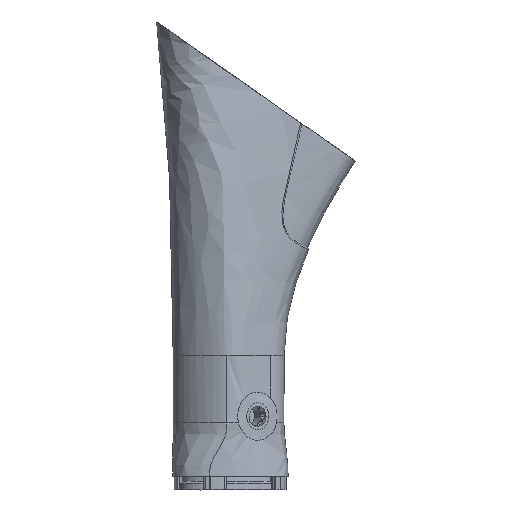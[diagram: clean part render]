
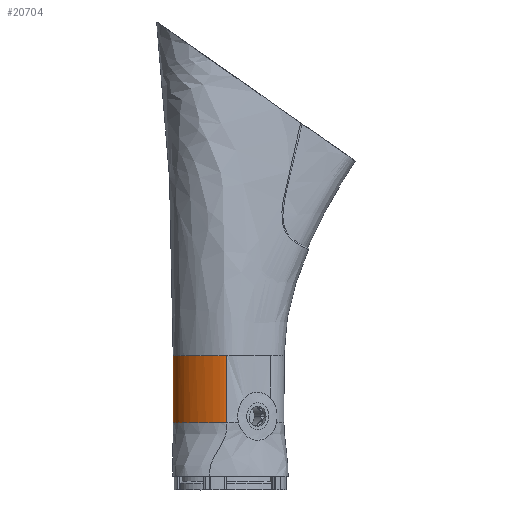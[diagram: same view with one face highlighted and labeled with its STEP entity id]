
A CAD part, left-side view. The second image highlights one B-rep face of the part: STEP entity #20704.
In plain terms, the highlighted free-form (B-spline) face has degree [3, 1] with [6, 2] control points.
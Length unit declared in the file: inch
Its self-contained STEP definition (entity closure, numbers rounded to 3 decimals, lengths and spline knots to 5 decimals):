
#194 = CARTESIAN_POINT ( 'NONE',  ( 0.05, 0.69, 1.5 ) ) ;
#334 = CARTESIAN_POINT ( 'NONE',  ( -0.89443, -0.31, 0.25 ) ) ;
#439 = CARTESIAN_POINT ( 'NONE',  ( 0.89443, -0.31, -3.73696 ) ) ;
#663 = ORIENTED_EDGE ( 'NONE', *, *, #16492, .F. ) ;
#770 = CARTESIAN_POINT ( 'NONE',  ( 0.89443, -0.31, 0.25 ) ) ;
#801 = CARTESIAN_POINT ( 'NONE',  ( 0.89443, -0.085, 0.25 ) ) ;
#976 = CARTESIAN_POINT ( 'NONE',  ( 0.89443, -0.085, 0.25 ) ) ;
#1501 = VERTEX_POINT ( 'NONE', #1584 ) ;
#1584 = CARTESIAN_POINT ( 'NONE',  ( 0.89443, -0.31, 1.5 ) ) ;
#1792 = DIRECTION ( 'NONE',  ( 0., 0., 1. ) ) ;
#2151 = LINE ( 'NONE', #5636, #6330 ) ;
#3338 = CARTESIAN_POINT ( 'NONE',  ( -0.89443, -0.31, 1.5 ) ) ;
#3463 = CARTESIAN_POINT ( 'NONE',  ( 0.89443, -0.31, 1.5 ) ) ;
#3648 = EDGE_CURVE ( 'NONE', #6380, #21719, #2151, .T. ) ;
#4115 = ORIENTED_EDGE ( 'NONE', *, *, #3648, .T. ) ;
#4367 = CARTESIAN_POINT ( 'NONE',  ( 0.51556, 0.69646, 0.25 ) ) ;
#5636 = CARTESIAN_POINT ( 'NONE',  ( -0.89443, -0.31, -3.73696 ) ) ;
#5839 = CARTESIAN_POINT ( 'NONE',  ( -0.89443, -0.31, 0.25 ) ) ;
#5906 = CARTESIAN_POINT ( 'NONE',  ( -0.55, 0.62542, 1.5 ) ) ;
#6310 = CARTESIAN_POINT ( 'NONE',  ( -0.89443, -0.085, 1.5 ) ) ;
#6330 = VECTOR ( 'NONE', #9129, 39.37008 ) ;
#6380 = VERTEX_POINT ( 'NONE', #334 ) ;
#6917 = EDGE_CURVE ( 'NONE', #1501, #19373, #16355, .T. ) ;
#7063 = CARTESIAN_POINT ( 'NONE',  ( 0., 0.69, 1.5 ) ) ;
#9067 = CARTESIAN_POINT ( 'NONE',  ( 0., 0.69, 1.5 ) ) ;
#9129 = DIRECTION ( 'NONE',  ( 0., 0., 1. ) ) ;
#9435 = EDGE_CURVE ( 'NONE', #19373, #21719, #16594, .T. ) ;
#10224 = CARTESIAN_POINT ( 'NONE',  ( 0.55, 0.62542, 1.5 ) ) ;
#11580 = ORIENTED_EDGE ( 'NONE', *, *, #16916, .F. ) ;
#11962 = VERTEX_POINT ( 'NONE', #14994 ) ;
#12453 = CARTESIAN_POINT ( 'NONE',  ( 0.89443, -0.31, 1.5 ) ) ;
#12692 = CARTESIAN_POINT ( 'NONE',  ( -0.89443, -0.085, 0.25 ) ) ;
#12907 = CARTESIAN_POINT ( 'NONE',  ( -0.51556, 0.69646, 0.25 ) ) ;
#13279 = CARTESIAN_POINT ( 'NONE',  ( -0.51556, 0.69646, 0.25 ) ) ;
#13825 = LINE ( 'NONE', #439, #17006 ) ;
#14020 = ORIENTED_EDGE ( 'NONE', *, *, #9435, .F. ) ;
#14145 = CARTESIAN_POINT ( 'NONE',  ( 0.89443, -0.31, 0.25 ) ) ;
#14547 = CARTESIAN_POINT ( 'NONE',  ( 0., 0.69, 1.5 ) ) ;
#14630 = CARTESIAN_POINT ( 'NONE',  ( -0.51556, 0.69646, 1.5 ) ) ;
#14847 = CARTESIAN_POINT ( 'NONE',  ( -0.89443, -0.31, 0.25 ) ) ;
#14961 = CARTESIAN_POINT ( 'NONE',  ( -0.89443, -0.31, 1.5 ) ) ;
#14994 = CARTESIAN_POINT ( 'NONE',  ( 0.89443, -0.31, 0.25 ) ) ;
#16023 = CARTESIAN_POINT ( 'NONE',  ( -0.89443, -0.31, 1.5 ) ) ;
#16205 = CARTESIAN_POINT ( 'NONE',  ( 0.51556, 0.69646, 1.5 ) ) ;
#16355 = B_SPLINE_CURVE_WITH_KNOTS ( 'NONE', 3,
 ( #3463, #22021, #10224, #194, #7063 ),
 .UNSPECIFIED., .F., .F.,
 ( 4, 1, 4 ),
 ( 0., 0.45, 0.5 ),
 .UNSPECIFIED. ) ;
#16492 = EDGE_CURVE ( 'NONE', #11962, #1501, #13825, .T. ) ;
#16594 = B_SPLINE_CURVE_WITH_KNOTS ( 'NONE', 3,
 ( #9067, #19175, #5906, #20871, #16023 ),
 .UNSPECIFIED., .F., .F.,
 ( 4, 1, 4 ),
 ( 0.5, 0.55, 1. ),
 .UNSPECIFIED. ) ;
#16916 = EDGE_CURVE ( 'NONE', #6380, #11962, #18131, .T. ) ;
#16967 = B_SPLINE_SURFACE_WITH_KNOTS ( 'NONE', 3, 1, ( 
 ( #14847, #14961 ),
 ( #21711, #6310 ),
 ( #13279, #14630 ),
 ( #20143, #16205 ),
 ( #801, #21009 ),
 ( #14145, #12453 ) ),
 .UNSPECIFIED., .F., .F., .F.,
 ( 4, 1, 1, 4 ),
 ( 2, 2 ),
 ( 0., 0.45, 0.55, 1. ),
 ( 0., 1. ),
 .UNSPECIFIED. ) ;
#17006 = VECTOR ( 'NONE', #1792, 39.37008 ) ;
#17616 = EDGE_LOOP ( 'NONE', ( #11580, #4115, #14020, #18070, #663 ) ) ;
#18070 = ORIENTED_EDGE ( 'NONE', *, *, #6917, .F. ) ;
#18131 = B_SPLINE_CURVE_WITH_KNOTS ( 'NONE', 3,
 ( #5839, #12692, #12907, #4367, #976, #770 ),
 .UNSPECIFIED., .F., .F.,
 ( 4, 1, 1, 4 ),
 ( 0., 0.45, 0.55, 1. ),
 .UNSPECIFIED. ) ;
#18336 = FACE_OUTER_BOUND ( 'NONE', #17616, .T. ) ;
#19175 = CARTESIAN_POINT ( 'NONE',  ( -0.05, 0.69, 1.5 ) ) ;
#19373 = VERTEX_POINT ( 'NONE', #14547 ) ;
#20143 = CARTESIAN_POINT ( 'NONE',  ( 0.51556, 0.69646, 0.25 ) ) ;
#20704 = ADVANCED_FACE ( 'NONE', ( #18336 ), #16967, .F. ) ;
#20871 = CARTESIAN_POINT ( 'NONE',  ( -0.89443, -0.085, 1.5 ) ) ;
#21009 = CARTESIAN_POINT ( 'NONE',  ( 0.89443, -0.085, 1.5 ) ) ;
#21711 = CARTESIAN_POINT ( 'NONE',  ( -0.89443, -0.085, 0.25 ) ) ;
#21719 = VERTEX_POINT ( 'NONE', #3338 ) ;
#22021 = CARTESIAN_POINT ( 'NONE',  ( 0.89443, -0.085, 1.5 ) ) ;
